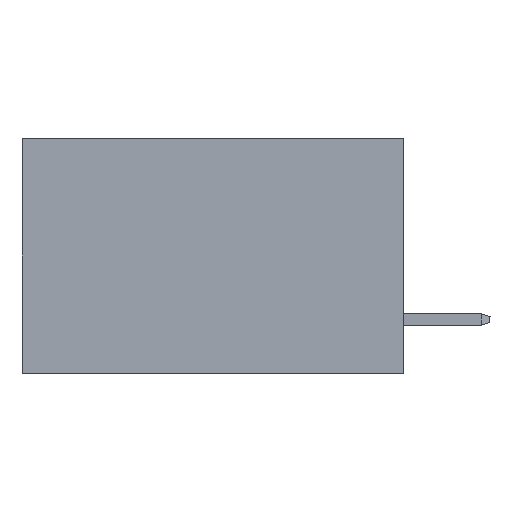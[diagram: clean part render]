
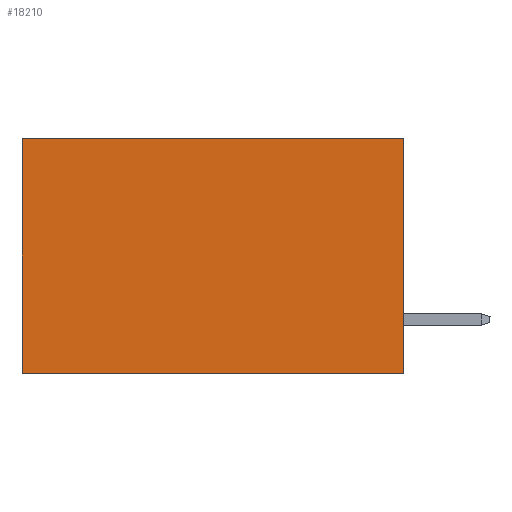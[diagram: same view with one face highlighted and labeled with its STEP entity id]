
A CAD part, left-side view. The second image highlights one B-rep face of the part: STEP entity #18210.
In plain terms, the highlighted planar face has unit normal (-1, 0, 0).
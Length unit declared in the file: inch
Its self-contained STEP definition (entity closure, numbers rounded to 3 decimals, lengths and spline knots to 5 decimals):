
#88 = CARTESIAN_POINT ( 'NONE',  ( 0.2875, 0., 0. ) ) ;
#1645 = VECTOR ( 'NONE', #12866, 39.37008 ) ;
#2477 = CARTESIAN_POINT ( 'NONE',  ( 0.2875, 0., 0. ) ) ;
#2775 = CARTESIAN_POINT ( 'NONE',  ( 0.2875, 0.6, 0. ) ) ;
#2815 = ORIENTED_EDGE ( 'NONE', *, *, #6725, .F. ) ;
#3709 = CARTESIAN_POINT ( 'NONE',  ( 0.2875, 0., 0. ) ) ;
#4306 = DIRECTION ( 'NONE',  ( 0., 0., -1. ) ) ;
#4331 = DIRECTION ( 'NONE',  ( 0., 1., 0. ) ) ;
#4602 = PLANE ( 'NONE',  #5117 ) ;
#5117 = AXIS2_PLACEMENT_3D ( 'NONE', #88, #16619, #4306 ) ;
#5697 = LINE ( 'NONE', #24238, #1645 ) ;
#6370 = CARTESIAN_POINT ( 'NONE',  ( 0.2875, 0., -0.37 ) ) ;
#6624 = ORIENTED_EDGE ( 'NONE', *, *, #27222, .T. ) ;
#6725 = EDGE_CURVE ( 'NONE', #15097, #7269, #21346, .T. ) ;
#7269 = VERTEX_POINT ( 'NONE', #29236 ) ;
#8198 = EDGE_CURVE ( 'NONE', #7269, #16287, #16032, .T. ) ;
#9035 = LINE ( 'NONE', #30221, #21873 ) ;
#11848 = EDGE_CURVE ( 'NONE', #25780, #16287, #9035, .T. ) ;
#12866 = DIRECTION ( 'NONE',  ( 0., 1., 0. ) ) ;
#13862 = DIRECTION ( 'NONE',  ( 0., 0., -1. ) ) ;
#15097 = VERTEX_POINT ( 'NONE', #3709 ) ;
#16032 = LINE ( 'NONE', #6370, #22304 ) ;
#16287 = VERTEX_POINT ( 'NONE', #17444 ) ;
#16619 = DIRECTION ( 'NONE',  ( 1., 0., 0. ) ) ;
#17444 = CARTESIAN_POINT ( 'NONE',  ( 0.2875, 0.6, -0.37 ) ) ;
#18210 = ADVANCED_FACE ( 'NONE', ( #18660 ), #4602, .F. ) ;
#18660 = FACE_OUTER_BOUND ( 'NONE', #23299, .T. ) ;
#21346 = LINE ( 'NONE', #2477, #26004 ) ;
#21873 = VECTOR ( 'NONE', #13862, 39.37008 ) ;
#22304 = VECTOR ( 'NONE', #4331, 39.37008 ) ;
#22413 = ORIENTED_EDGE ( 'NONE', *, *, #11848, .T. ) ;
#23299 = EDGE_LOOP ( 'NONE', ( #22413, #30797, #2815, #6624 ) ) ;
#24238 = CARTESIAN_POINT ( 'NONE',  ( 0.2875, 0., 0. ) ) ;
#25780 = VERTEX_POINT ( 'NONE', #2775 ) ;
#26004 = VECTOR ( 'NONE', #26462, 39.37008 ) ;
#26462 = DIRECTION ( 'NONE',  ( 0., 0., -1. ) ) ;
#27222 = EDGE_CURVE ( 'NONE', #15097, #25780, #5697, .T. ) ;
#29236 = CARTESIAN_POINT ( 'NONE',  ( 0.2875, 0., -0.37 ) ) ;
#30221 = CARTESIAN_POINT ( 'NONE',  ( 0.2875, 0.6, 0. ) ) ;
#30797 = ORIENTED_EDGE ( 'NONE', *, *, #8198, .F. ) ;
